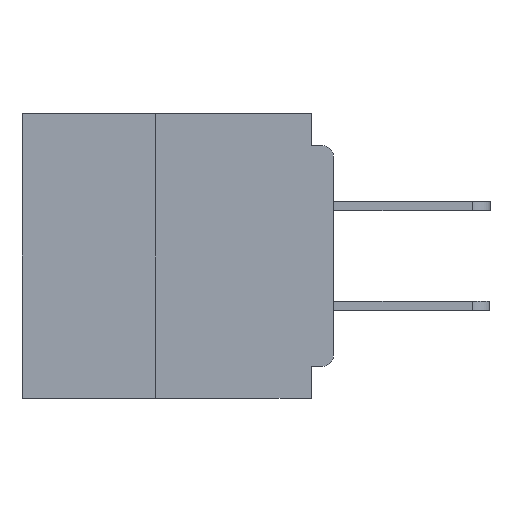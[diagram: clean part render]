
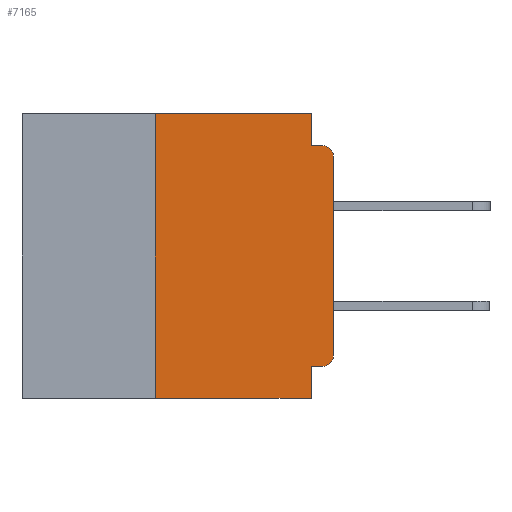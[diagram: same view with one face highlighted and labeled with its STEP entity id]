
A CAD part, left-side view. The second image highlights one B-rep face of the part: STEP entity #7165.
In plain terms, the highlighted planar face has unit normal (-1, 0, 0).
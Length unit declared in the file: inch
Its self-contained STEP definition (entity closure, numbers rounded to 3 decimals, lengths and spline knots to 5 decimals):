
#49 = ORIENTED_EDGE ( 'NONE', *, *, #33484, .F. ) ;
#811 = DIRECTION ( 'NONE',  ( 1., 0., 0. ) ) ;
#834 = VERTEX_POINT ( 'NONE', #15482 ) ;
#1374 = CARTESIAN_POINT ( 'NONE',  ( 0., 0.437, -0.4 ) ) ;
#1719 = CARTESIAN_POINT ( 'NONE',  ( 0., 0., -0.355 ) ) ;
#2122 = ORIENTED_EDGE ( 'NONE', *, *, #13169, .F. ) ;
#2192 = VERTEX_POINT ( 'NONE', #33301 ) ;
#2476 = DIRECTION ( 'NONE',  ( 0., -1., 0. ) ) ;
#2725 = VECTOR ( 'NONE', #6177, 39.37008 ) ;
#4024 = VERTEX_POINT ( 'NONE', #11993 ) ;
#4026 = CIRCLE ( 'NONE', #13831, 0.015 ) ;
#5604 = ORIENTED_EDGE ( 'NONE', *, *, #21749, .T. ) ;
#5880 = VECTOR ( 'NONE', #36141, 39.37008 ) ;
#6177 = DIRECTION ( 'NONE',  ( 0., 0., 1. ) ) ;
#6206 = VERTEX_POINT ( 'NONE', #16163 ) ;
#6522 = ORIENTED_EDGE ( 'NONE', *, *, #8708, .F. ) ;
#7165 = ADVANCED_FACE ( 'NONE', ( #10553 ), #34986, .F. ) ;
#7187 = ORIENTED_EDGE ( 'NONE', *, *, #20300, .F. ) ;
#7235 = ORIENTED_EDGE ( 'NONE', *, *, #18426, .T. ) ;
#7975 = ORIENTED_EDGE ( 'NONE', *, *, #11576, .T. ) ;
#8708 = EDGE_CURVE ( 'NONE', #4024, #28416, #26061, .T. ) ;
#8997 = VECTOR ( 'NONE', #27126, 39.37008 ) ;
#9398 = EDGE_CURVE ( 'NONE', #15348, #2192, #12200, .T. ) ;
#10553 = FACE_OUTER_BOUND ( 'NONE', #17510, .T. ) ;
#11299 = EDGE_CURVE ( 'NONE', #18510, #34428, #28142, .T. ) ;
#11526 = ORIENTED_EDGE ( 'NONE', *, *, #16407, .F. ) ;
#11576 = EDGE_CURVE ( 'NONE', #4024, #15348, #4026, .T. ) ;
#11993 = CARTESIAN_POINT ( 'NONE',  ( 0., 0.015, -0.355 ) ) ;
#12200 = LINE ( 'NONE', #34538, #2725 ) ;
#12868 = DIRECTION ( 'NONE',  ( 0., -1., 0. ) ) ;
#13169 = EDGE_CURVE ( 'NONE', #28416, #30446, #16669, .T. ) ;
#13568 = VERTEX_POINT ( 'NONE', #28851 ) ;
#13831 = AXIS2_PLACEMENT_3D ( 'NONE', #16105, #35841, #19001 ) ;
#14427 = LINE ( 'NONE', #16436, #5880 ) ;
#14510 = VECTOR ( 'NONE', #12868, 39.37008 ) ;
#14891 = DIRECTION ( 'NONE',  ( -1., 0., 0. ) ) ;
#15006 = CARTESIAN_POINT ( 'NONE',  ( 0., 0.437, 0. ) ) ;
#15064 = AXIS2_PLACEMENT_3D ( 'NONE', #31872, #14891, #34660 ) ;
#15348 = VERTEX_POINT ( 'NONE', #22075 ) ;
#15482 = CARTESIAN_POINT ( 'NONE',  ( 0., 0.031, -0.045 ) ) ;
#16105 = CARTESIAN_POINT ( 'NONE',  ( 0., 0.015, -0.34 ) ) ;
#16163 = CARTESIAN_POINT ( 'NONE',  ( 0., 0.015, -0.045 ) ) ;
#16315 = LINE ( 'NONE', #1374, #14510 ) ;
#16407 = EDGE_CURVE ( 'NONE', #34428, #834, #22200, .T. ) ;
#16436 = CARTESIAN_POINT ( 'NONE',  ( 0., 0.25, -0.4 ) ) ;
#16498 = LINE ( 'NONE', #16897, #30658 ) ;
#16565 = CIRCLE ( 'NONE', #15064, 0.015 ) ;
#16669 = LINE ( 'NONE', #32817, #8997 ) ;
#16897 = CARTESIAN_POINT ( 'NONE',  ( 0., 0., -0.045 ) ) ;
#17510 = EDGE_LOOP ( 'NONE', ( #33125, #5604, #49, #11526, #29407, #7187, #7235, #2122, #6522, #7975 ) ) ;
#18124 = CARTESIAN_POINT ( 'NONE',  ( 0., 0.437, 0. ) ) ;
#18371 = CARTESIAN_POINT ( 'NONE',  ( 0., 0.031, -0.355 ) ) ;
#18426 = EDGE_CURVE ( 'NONE', #13568, #30446, #16315, .T. ) ;
#18510 = VERTEX_POINT ( 'NONE', #30414 ) ;
#18661 = DIRECTION ( 'NONE',  ( 0., 0., -1. ) ) ;
#19001 = DIRECTION ( 'NONE',  ( 0., 0., -1. ) ) ;
#20300 = EDGE_CURVE ( 'NONE', #13568, #18510, #14427, .T. ) ;
#20995 = DIRECTION ( 'NONE',  ( 0., 0., -1. ) ) ;
#21536 = VECTOR ( 'NONE', #31993, 39.37008 ) ;
#21749 = EDGE_CURVE ( 'NONE', #2192, #6206, #16565, .T. ) ;
#22075 = CARTESIAN_POINT ( 'NONE',  ( 0., 0., -0.34 ) ) ;
#22200 = LINE ( 'NONE', #35505, #23072 ) ;
#23072 = VECTOR ( 'NONE', #18661, 39.37008 ) ;
#24964 = CARTESIAN_POINT ( 'NONE',  ( 0., 0.031, -0.4 ) ) ;
#25171 = VECTOR ( 'NONE', #35860, 39.37008 ) ;
#26061 = LINE ( 'NONE', #1719, #25171 ) ;
#27126 = DIRECTION ( 'NONE',  ( 0., 0., -1. ) ) ;
#27339 = CARTESIAN_POINT ( 'NONE',  ( 0., 0.031, 0. ) ) ;
#28142 = LINE ( 'NONE', #15006, #21536 ) ;
#28416 = VERTEX_POINT ( 'NONE', #18371 ) ;
#28851 = CARTESIAN_POINT ( 'NONE',  ( 0., 0.25, -0.4 ) ) ;
#29407 = ORIENTED_EDGE ( 'NONE', *, *, #11299, .F. ) ;
#30414 = CARTESIAN_POINT ( 'NONE',  ( 0., 0.25, 0. ) ) ;
#30446 = VERTEX_POINT ( 'NONE', #24964 ) ;
#30658 = VECTOR ( 'NONE', #2476, 39.37008 ) ;
#31872 = CARTESIAN_POINT ( 'NONE',  ( 0., 0.015, -0.06 ) ) ;
#31993 = DIRECTION ( 'NONE',  ( 0., -1., 0. ) ) ;
#32817 = CARTESIAN_POINT ( 'NONE',  ( 0., 0.031, -0.4 ) ) ;
#33125 = ORIENTED_EDGE ( 'NONE', *, *, #9398, .T. ) ;
#33301 = CARTESIAN_POINT ( 'NONE',  ( 0., 0., -0.06 ) ) ;
#33484 = EDGE_CURVE ( 'NONE', #834, #6206, #16498, .T. ) ;
#34428 = VERTEX_POINT ( 'NONE', #27339 ) ;
#34538 = CARTESIAN_POINT ( 'NONE',  ( 0., 0., 0. ) ) ;
#34660 = DIRECTION ( 'NONE',  ( 0., 0., -1. ) ) ;
#34986 = PLANE ( 'NONE',  #35295 ) ;
#35295 = AXIS2_PLACEMENT_3D ( 'NONE', #18124, #811, #20995 ) ;
#35505 = CARTESIAN_POINT ( 'NONE',  ( 0., 0.031, 0. ) ) ;
#35841 = DIRECTION ( 'NONE',  ( -1., 0., 0. ) ) ;
#35860 = DIRECTION ( 'NONE',  ( 0., 1., 0. ) ) ;
#36141 = DIRECTION ( 'NONE',  ( 0., 0., 1. ) ) ;
